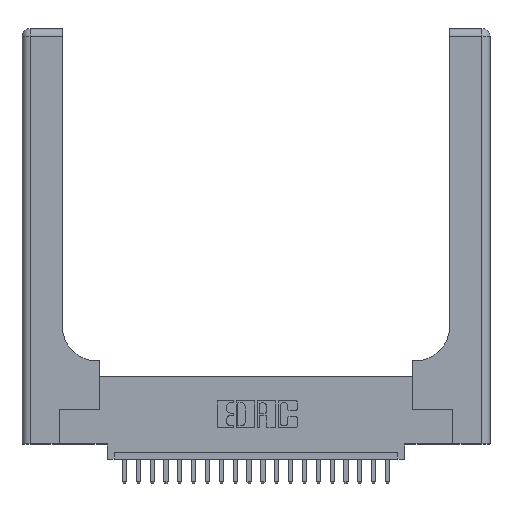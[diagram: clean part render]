
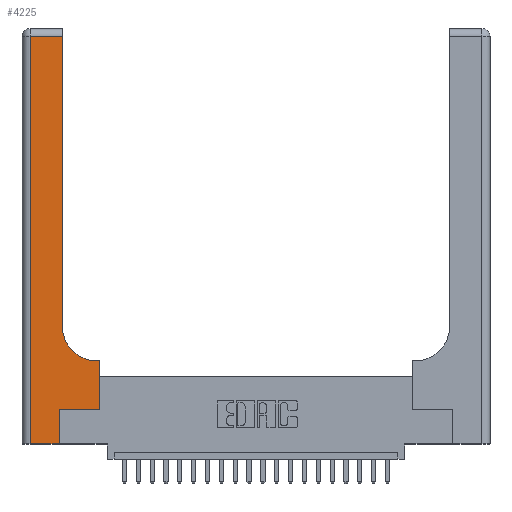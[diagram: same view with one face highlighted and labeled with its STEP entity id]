
A CAD part, top view. The second image highlights one B-rep face of the part: STEP entity #4225.
In plain terms, the highlighted planar face has unit normal (0, 0, 1).
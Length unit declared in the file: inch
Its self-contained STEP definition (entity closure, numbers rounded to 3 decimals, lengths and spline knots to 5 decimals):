
#235 = DIRECTION ( 'NONE',  ( 0., 1., 0. ) ) ;
#694 = LINE ( 'NONE', #837, #5531 ) ;
#837 = CARTESIAN_POINT ( 'NONE',  ( 0.2915, 3., 0.37 ) ) ;
#1376 = DIRECTION ( 'NONE',  ( -1., 0., 0. ) ) ;
#1748 = ORIENTED_EDGE ( 'NONE', *, *, #6686, .T. ) ;
#2165 = ORIENTED_EDGE ( 'NONE', *, *, #16982, .T. ) ;
#2340 = LINE ( 'NONE', #21251, #20165 ) ;
#2439 = VERTEX_POINT ( 'NONE', #22823 ) ;
#3181 = CARTESIAN_POINT ( 'NONE',  ( 0.2915, 0.85, 0.37 ) ) ;
#3207 = DIRECTION ( 'NONE',  ( 0., 1., 0. ) ) ;
#3310 = EDGE_CURVE ( 'NONE', #16734, #19837, #23247, .T. ) ;
#3313 = VECTOR ( 'NONE', #235, 39.37008 ) ;
#3465 = DIRECTION ( 'NONE',  ( -1., 0., 0. ) ) ;
#4131 = VECTOR ( 'NONE', #3207, 39.37008 ) ;
#4185 = CARTESIAN_POINT ( 'NONE',  ( 0.5585, 0.25, 0.37 ) ) ;
#4225 = ADVANCED_FACE ( 'NONE', ( #11341 ), #13234, .F. ) ;
#4307 = ORIENTED_EDGE ( 'NONE', *, *, #21811, .T. ) ;
#4632 = CIRCLE ( 'NONE', #8195, 0.25 ) ;
#4882 = EDGE_CURVE ( 'NONE', #15749, #15853, #11585, .T. ) ;
#5012 = DIRECTION ( 'NONE',  ( 0., -1., 0. ) ) ;
#5527 = LINE ( 'NONE', #15284, #19369 ) ;
#5531 = VECTOR ( 'NONE', #13523, 39.37008 ) ;
#5625 = CARTESIAN_POINT ( 'NONE',  ( 0.5585, 0.25, 0.37 ) ) ;
#6097 = EDGE_CURVE ( 'NONE', #23231, #19760, #14901, .T. ) ;
#6398 = DIRECTION ( 'NONE',  ( 0., 0., -1. ) ) ;
#6657 = LINE ( 'NONE', #16390, #21682 ) ;
#6686 = EDGE_CURVE ( 'NONE', #22530, #16734, #694, .T. ) ;
#8195 = AXIS2_PLACEMENT_3D ( 'NONE', #17224, #6398, #20568 ) ;
#8323 = AXIS2_PLACEMENT_3D ( 'NONE', #15192, #16977, #15336 ) ;
#8560 = CARTESIAN_POINT ( 'NONE',  ( 0.06, 3., 0.37 ) ) ;
#9058 = CARTESIAN_POINT ( 'NONE',  ( 0.269, 0., 0.37 ) ) ;
#10291 = CARTESIAN_POINT ( 'NONE',  ( 0.5585, 0.6, 0.37 ) ) ;
#10645 = VECTOR ( 'NONE', #5012, 39.37008 ) ;
#11145 = VERTEX_POINT ( 'NONE', #14350 ) ;
#11341 = FACE_OUTER_BOUND ( 'NONE', #13301, .T. ) ;
#11585 = LINE ( 'NONE', #5625, #3313 ) ;
#12734 = ORIENTED_EDGE ( 'NONE', *, *, #17823, .T. ) ;
#13054 = ORIENTED_EDGE ( 'NONE', *, *, #6097, .T. ) ;
#13234 = PLANE ( 'NONE',  #8323 ) ;
#13301 = EDGE_LOOP ( 'NONE', ( #1748, #18337, #2165, #17236, #13054, #12734, #21395, #14302, #4307 ) ) ;
#13523 = DIRECTION ( 'NONE',  ( 0., 1., 0. ) ) ;
#13794 = CARTESIAN_POINT ( 'NONE',  ( 0.06, 2.94, 0.37 ) ) ;
#14302 = ORIENTED_EDGE ( 'NONE', *, *, #22632, .T. ) ;
#14350 = CARTESIAN_POINT ( 'NONE',  ( 0.06, 0., 0.37 ) ) ;
#14825 = CARTESIAN_POINT ( 'NONE',  ( 0., 2.94, 0.37 ) ) ;
#14901 = LINE ( 'NONE', #21196, #4131 ) ;
#14922 = CARTESIAN_POINT ( 'NONE',  ( 0.2915, 2.94, 0.37 ) ) ;
#15192 = CARTESIAN_POINT ( 'NONE',  ( 0., 3., 0.37 ) ) ;
#15284 = CARTESIAN_POINT ( 'NONE',  ( 0.269, 0.25, 0.37 ) ) ;
#15336 = DIRECTION ( 'NONE',  ( -1., 0., 0. ) ) ;
#15749 = VERTEX_POINT ( 'NONE', #4185 ) ;
#15853 = VERTEX_POINT ( 'NONE', #10291 ) ;
#16390 = CARTESIAN_POINT ( 'NONE',  ( 0., 0., 0.37 ) ) ;
#16734 = VERTEX_POINT ( 'NONE', #14922 ) ;
#16928 = DIRECTION ( 'NONE',  ( 1., 0., 0. ) ) ;
#16977 = DIRECTION ( 'NONE',  ( 0., 0., -1. ) ) ;
#16982 = EDGE_CURVE ( 'NONE', #19837, #11145, #20796, .T. ) ;
#17157 = CARTESIAN_POINT ( 'NONE',  ( 0.269, 0.25, 0.37 ) ) ;
#17224 = CARTESIAN_POINT ( 'NONE',  ( 0.5415, 0.85, 0.37 ) ) ;
#17236 = ORIENTED_EDGE ( 'NONE', *, *, #17290, .T. ) ;
#17290 = EDGE_CURVE ( 'NONE', #11145, #23231, #6657, .T. ) ;
#17823 = EDGE_CURVE ( 'NONE', #19760, #15749, #5527, .T. ) ;
#18337 = ORIENTED_EDGE ( 'NONE', *, *, #3310, .T. ) ;
#18429 = VECTOR ( 'NONE', #3465, 39.37008 ) ;
#19369 = VECTOR ( 'NONE', #16928, 39.37008 ) ;
#19760 = VERTEX_POINT ( 'NONE', #17157 ) ;
#19837 = VERTEX_POINT ( 'NONE', #13794 ) ;
#20165 = VECTOR ( 'NONE', #1376, 39.37008 ) ;
#20188 = DIRECTION ( 'NONE',  ( 1., 0., 0. ) ) ;
#20568 = DIRECTION ( 'NONE',  ( 1., 0., 0. ) ) ;
#20796 = LINE ( 'NONE', #8560, #10645 ) ;
#21196 = CARTESIAN_POINT ( 'NONE',  ( 0.269, 0., 0.37 ) ) ;
#21251 = CARTESIAN_POINT ( 'NONE',  ( 0.2915, 0.6, 0.37 ) ) ;
#21395 = ORIENTED_EDGE ( 'NONE', *, *, #4882, .T. ) ;
#21682 = VECTOR ( 'NONE', #20188, 39.37008 ) ;
#21811 = EDGE_CURVE ( 'NONE', #2439, #22530, #4632, .T. ) ;
#22530 = VERTEX_POINT ( 'NONE', #3181 ) ;
#22632 = EDGE_CURVE ( 'NONE', #15853, #2439, #2340, .T. ) ;
#22823 = CARTESIAN_POINT ( 'NONE',  ( 0.5415, 0.6, 0.37 ) ) ;
#23231 = VERTEX_POINT ( 'NONE', #9058 ) ;
#23247 = LINE ( 'NONE', #14825, #18429 ) ;
